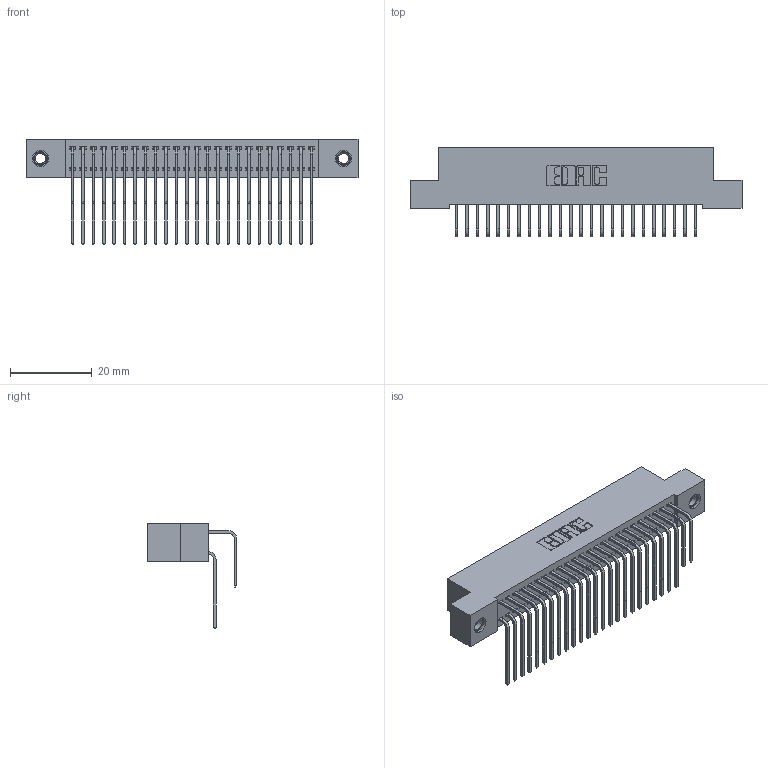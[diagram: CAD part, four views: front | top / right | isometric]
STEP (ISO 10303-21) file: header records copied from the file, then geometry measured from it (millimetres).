
FILE_DESCRIPTION (( 'STEP AP203' ), '1' );
FILE_NAME ('342-048-558-207.STEP', '2018-08-12T18:27:39', ( '' ), ( '' ), 'SwSTEP 2.0', 'SolidWorks 2016', '' );
FILE_SCHEMA (( 'CONFIG_CONTROL_DESIGN' ));
Length unit declared in the file: inch
Products named in the file (5): 345-250-001_345-250-005-103; 342-048-558-207; 342 Part_TI; 345-292-001_558 559 Tail - 1; 345-292-001_558 Tail - 2
Assembly tree (51 placements, depth 2):
  342-048-558-207
    342 Part_TI
    345-292-001_558 559 Tail - 1  x24
    345-292-001_558 Tail - 2  x24
    345-250-001_345-250-005-103  x2
Bounding box: 81.28 x 21.91 x 25.78 mm (x, y, z)
Volume: 7482 mm3; surface area: 13013.7 mm2
Topology: 51 solids, 51 shells, 2762 faces, 8163 edges, 5370 vertices
Faces by surface type: plane 1922, cylinder 824, cone 12, torus 4
Entity records: 20606 total; most frequent: CARTESIAN_POINT 3468, ORIENTED_EDGE 3346, DIRECTION 3007, EDGE_CURVE 1673, VECTOR 1485, LINE 1485, VERTEX_POINT 1108, AXIS2_PLACEMENT_3D 761
